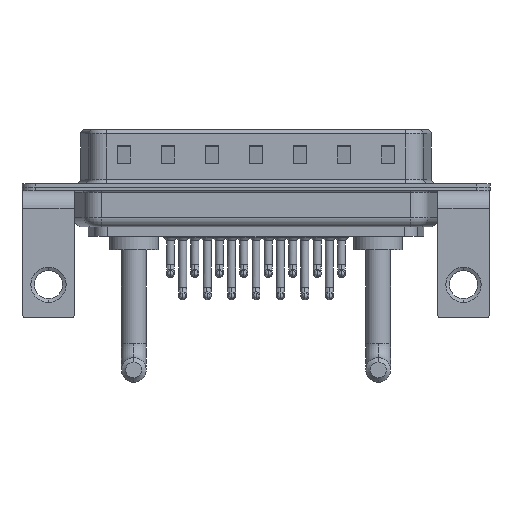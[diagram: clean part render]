
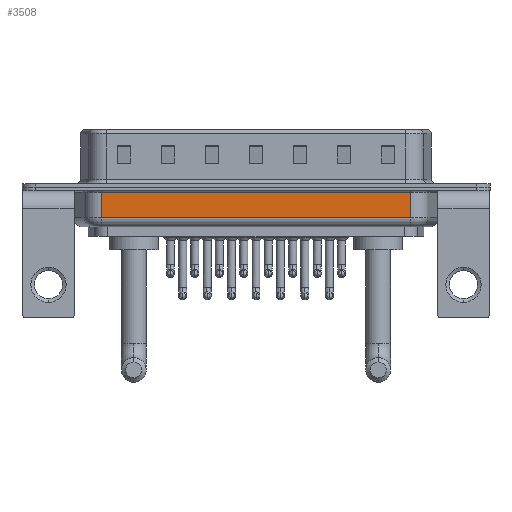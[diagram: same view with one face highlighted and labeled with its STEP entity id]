
A CAD part, front view. The second image highlights one B-rep face of the part: STEP entity #3508.
In plain terms, the highlighted planar face has unit normal (0, -1, 0).
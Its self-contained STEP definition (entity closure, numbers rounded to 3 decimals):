
#980 = ORIENTED_EDGE ( 'NONE', *, *, #8668, .T. ) ;
#1098 = VECTOR ( 'NONE', #11971, 1000. ) ;
#1571 = DIRECTION ( 'NONE',  ( -1., 0., 0. ) ) ;
#2124 = EDGE_CURVE ( 'NONE', #18226, #8350, #7123, .T. ) ;
#2748 = VECTOR ( 'NONE', #1571, 1000. ) ;
#3383 = CARTESIAN_POINT ( 'NONE',  ( 6.006, -5.35, -0.65 ) ) ;
#3508 = ADVANCED_FACE ( 'NONE', ( #17445 ), #19508, .F. ) ;
#5339 = AXIS2_PLACEMENT_3D ( 'NONE', #7648, #15631, #11627 ) ;
#6083 = VERTEX_POINT ( 'NONE', #11864 ) ;
#6241 = LINE ( 'NONE', #8179, #9526 ) ;
#7123 = LINE ( 'NONE', #3383, #2748 ) ;
#7648 = CARTESIAN_POINT ( 'NONE',  ( 6.006, -5.35, -4.5 ) ) ;
#8100 = CARTESIAN_POINT ( 'NONE',  ( 6.006, -5.35, -4.5 ) ) ;
#8179 = CARTESIAN_POINT ( 'NONE',  ( 6.006, -5.35, -3.5 ) ) ;
#8350 = VERTEX_POINT ( 'NONE', #14672 ) ;
#8668 = EDGE_CURVE ( 'NONE', #6083, #18226, #14617, .T. ) ;
#9034 = CARTESIAN_POINT ( 'NONE',  ( 41.044, -5.35, -0.65 ) ) ;
#9526 = VECTOR ( 'NONE', #16050, 1000. ) ;
#11509 = EDGE_CURVE ( 'NONE', #22561, #8350, #23326, .T. ) ;
#11627 = DIRECTION ( 'NONE',  ( 0., 0., 1. ) ) ;
#11864 = CARTESIAN_POINT ( 'NONE',  ( 41.044, -5.35, -3.5 ) ) ;
#11971 = DIRECTION ( 'NONE',  ( 0., 0., 1. ) ) ;
#13745 = ORIENTED_EDGE ( 'NONE', *, *, #19507, .T. ) ;
#14617 = LINE ( 'NONE', #24290, #22455 ) ;
#14672 = CARTESIAN_POINT ( 'NONE',  ( 6.006, -5.35, -0.65 ) ) ;
#15631 = DIRECTION ( 'NONE',  ( 0., 1., 0. ) ) ;
#16050 = DIRECTION ( 'NONE',  ( 1., 0., 0. ) ) ;
#17445 = FACE_OUTER_BOUND ( 'NONE', #25278, .T. ) ;
#18226 = VERTEX_POINT ( 'NONE', #9034 ) ;
#19177 = ORIENTED_EDGE ( 'NONE', *, *, #11509, .F. ) ;
#19507 = EDGE_CURVE ( 'NONE', #22561, #6083, #6241, .T. ) ;
#19508 = PLANE ( 'NONE',  #5339 ) ;
#21695 = CARTESIAN_POINT ( 'NONE',  ( 6.006, -5.35, -3.5 ) ) ;
#22455 = VECTOR ( 'NONE', #24032, 1000. ) ;
#22561 = VERTEX_POINT ( 'NONE', #21695 ) ;
#23326 = LINE ( 'NONE', #8100, #1098 ) ;
#23705 = ORIENTED_EDGE ( 'NONE', *, *, #2124, .T. ) ;
#24032 = DIRECTION ( 'NONE',  ( 0., 0., 1. ) ) ;
#24290 = CARTESIAN_POINT ( 'NONE',  ( 41.044, -5.35, -4.5 ) ) ;
#25278 = EDGE_LOOP ( 'NONE', ( #19177, #13745, #980, #23705 ) ) ;
